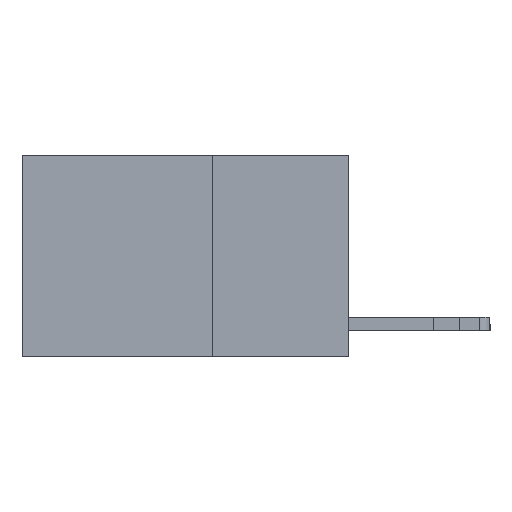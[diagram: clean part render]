
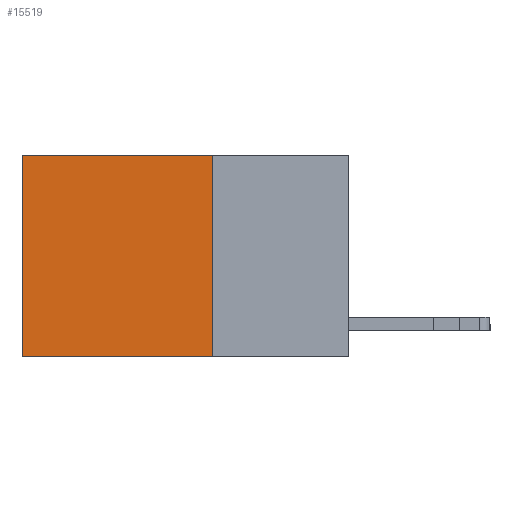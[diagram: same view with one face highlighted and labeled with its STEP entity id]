
A CAD part, left-side view. The second image highlights one B-rep face of the part: STEP entity #15519.
In plain terms, the highlighted planar face has unit normal (-1, 0, 0).
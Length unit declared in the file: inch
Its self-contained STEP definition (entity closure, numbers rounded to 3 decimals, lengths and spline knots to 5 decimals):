
#232 = EDGE_CURVE ( 'NONE', #14569, #16616, #1964, .T. ) ;
#378 = CARTESIAN_POINT ( 'NONE',  ( 0.2625, 0.25, 0. ) ) ;
#1438 = CARTESIAN_POINT ( 'NONE',  ( 0.2625, 0.6, -0.37 ) ) ;
#1579 = VECTOR ( 'NONE', #16040, 39.37008 ) ;
#1964 = LINE ( 'NONE', #378, #6381 ) ;
#3172 = LINE ( 'NONE', #9804, #1579 ) ;
#4394 = CARTESIAN_POINT ( 'NONE',  ( 0.2625, 0.6, 0. ) ) ;
#5137 = VERTEX_POINT ( 'NONE', #20690 ) ;
#6381 = VECTOR ( 'NONE', #19713, 39.37008 ) ;
#7174 = PLANE ( 'NONE',  #8086 ) ;
#7360 = EDGE_CURVE ( 'NONE', #16616, #18063, #20482, .T. ) ;
#7410 = DIRECTION ( 'NONE',  ( 0., 0., -1. ) ) ;
#8086 = AXIS2_PLACEMENT_3D ( 'NONE', #16590, #8343, #16492 ) ;
#8343 = DIRECTION ( 'NONE',  ( 1., 0., 0. ) ) ;
#8902 = VECTOR ( 'NONE', #19315, 39.37008 ) ;
#9271 = CARTESIAN_POINT ( 'NONE',  ( 0.2625, 0.25, 0. ) ) ;
#9804 = CARTESIAN_POINT ( 'NONE',  ( 0.2625, 0.25, -0.37 ) ) ;
#10042 = FACE_OUTER_BOUND ( 'NONE', #14097, .T. ) ;
#11614 = ORIENTED_EDGE ( 'NONE', *, *, #7360, .T. ) ;
#11730 = VECTOR ( 'NONE', #7410, 39.37008 ) ;
#12545 = CARTESIAN_POINT ( 'NONE',  ( 0.2625, 0.6, 0. ) ) ;
#13758 = ORIENTED_EDGE ( 'NONE', *, *, #20008, .F. ) ;
#14097 = EDGE_LOOP ( 'NONE', ( #11614, #16724, #13758, #20586 ) ) ;
#14569 = VERTEX_POINT ( 'NONE', #9271 ) ;
#15519 = ADVANCED_FACE ( 'NONE', ( #10042 ), #7174, .F. ) ;
#16040 = DIRECTION ( 'NONE',  ( 0., 1., 0. ) ) ;
#16492 = DIRECTION ( 'NONE',  ( 0., 0., -1. ) ) ;
#16590 = CARTESIAN_POINT ( 'NONE',  ( 0.2625, 0.25, 0. ) ) ;
#16616 = VERTEX_POINT ( 'NONE', #4394 ) ;
#16724 = ORIENTED_EDGE ( 'NONE', *, *, #19461, .F. ) ;
#16825 = CARTESIAN_POINT ( 'NONE',  ( 0.2625, 0.25, 0. ) ) ;
#18063 = VERTEX_POINT ( 'NONE', #1438 ) ;
#19315 = DIRECTION ( 'NONE',  ( 0., 0., -1. ) ) ;
#19461 = EDGE_CURVE ( 'NONE', #5137, #18063, #3172, .T. ) ;
#19713 = DIRECTION ( 'NONE',  ( 0., 1., 0. ) ) ;
#20008 = EDGE_CURVE ( 'NONE', #14569, #5137, #20322, .T. ) ;
#20322 = LINE ( 'NONE', #16825, #11730 ) ;
#20482 = LINE ( 'NONE', #12545, #8902 ) ;
#20586 = ORIENTED_EDGE ( 'NONE', *, *, #232, .T. ) ;
#20690 = CARTESIAN_POINT ( 'NONE',  ( 0.2625, 0.25, -0.37 ) ) ;
